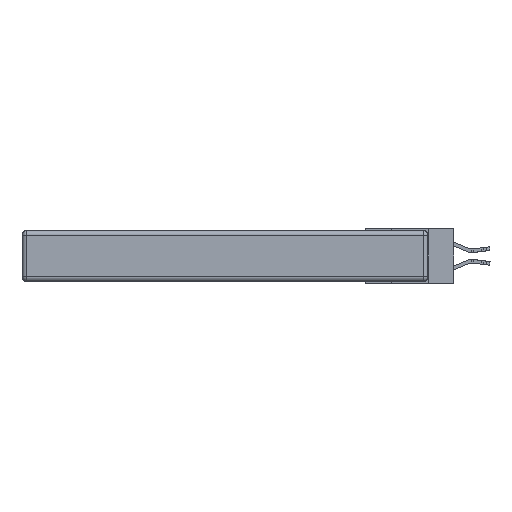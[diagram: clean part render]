
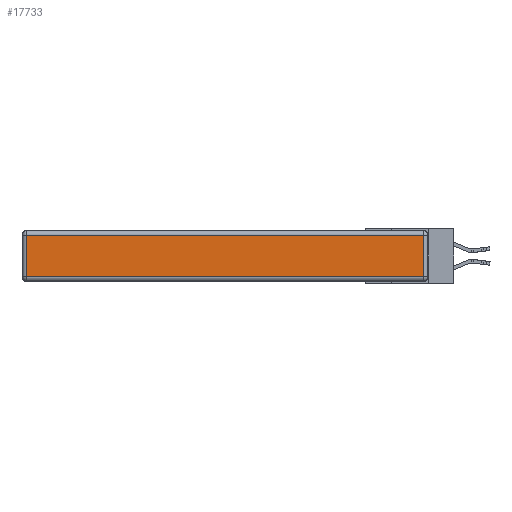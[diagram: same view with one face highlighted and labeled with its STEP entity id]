
A CAD part, left-side view. The second image highlights one B-rep face of the part: STEP entity #17733.
In plain terms, the highlighted planar face has unit normal (-1, 0, 0).
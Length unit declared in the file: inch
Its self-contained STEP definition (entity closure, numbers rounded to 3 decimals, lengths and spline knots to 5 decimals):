
#288 = LINE ( 'NONE', #23398, #34174 ) ;
#1447 = LINE ( 'NONE', #11361, #13348 ) ;
#2224 = PLANE ( 'NONE',  #32942 ) ;
#2473 = EDGE_CURVE ( 'NONE', #10716, #35085, #288, .T. ) ;
#3877 = CARTESIAN_POINT ( 'NONE',  ( 0., 2.72, -0.03 ) ) ;
#3889 = ORIENTED_EDGE ( 'NONE', *, *, #24011, .T. ) ;
#5048 = VECTOR ( 'NONE', #9613, 39.37008 ) ;
#6638 = CARTESIAN_POINT ( 'NONE',  ( 0., 0.03, -0.343 ) ) ;
#7925 = VERTEX_POINT ( 'NONE', #21688 ) ;
#8043 = VERTEX_POINT ( 'NONE', #25002 ) ;
#9613 = DIRECTION ( 'NONE',  ( 0., 0., 1. ) ) ;
#9906 = DIRECTION ( 'NONE',  ( 0., -1., 0. ) ) ;
#10716 = VERTEX_POINT ( 'NONE', #3877 ) ;
#10955 = FACE_OUTER_BOUND ( 'NONE', #35628, .T. ) ;
#11361 = CARTESIAN_POINT ( 'NONE',  ( 0., 2.75, -0.03 ) ) ;
#13348 = VECTOR ( 'NONE', #14070, 39.37008 ) ;
#13727 = ORIENTED_EDGE ( 'NONE', *, *, #20239, .T. ) ;
#14070 = DIRECTION ( 'NONE',  ( 0., 1., 0. ) ) ;
#15763 = DIRECTION ( 'NONE',  ( -1., 0., 0. ) ) ;
#17733 = ADVANCED_FACE ( 'NONE', ( #10955 ), #2224, .T. ) ;
#18973 = CARTESIAN_POINT ( 'NONE',  ( 0., 0., -0.343 ) ) ;
#20239 = EDGE_CURVE ( 'NONE', #7925, #10716, #1447, .T. ) ;
#21597 = EDGE_CURVE ( 'NONE', #35085, #8043, #23354, .T. ) ;
#21688 = CARTESIAN_POINT ( 'NONE',  ( 0., 0.03, -0.03 ) ) ;
#21885 = ORIENTED_EDGE ( 'NONE', *, *, #21597, .T. ) ;
#23354 = LINE ( 'NONE', #32181, #35647 ) ;
#23398 = CARTESIAN_POINT ( 'NONE',  ( 0., 2.72, -0.343 ) ) ;
#24011 = EDGE_CURVE ( 'NONE', #8043, #7925, #35017, .T. ) ;
#24137 = DIRECTION ( 'NONE',  ( 0., 0., 1. ) ) ;
#25002 = CARTESIAN_POINT ( 'NONE',  ( 0., 0.03, -0.313 ) ) ;
#25596 = DIRECTION ( 'NONE',  ( 0., 0., -1. ) ) ;
#29970 = ORIENTED_EDGE ( 'NONE', *, *, #2473, .T. ) ;
#32181 = CARTESIAN_POINT ( 'NONE',  ( 0., 0., -0.313 ) ) ;
#32942 = AXIS2_PLACEMENT_3D ( 'NONE', #18973, #15763, #24137 ) ;
#33662 = CARTESIAN_POINT ( 'NONE',  ( 0., 2.72, -0.313 ) ) ;
#34174 = VECTOR ( 'NONE', #25596, 39.37008 ) ;
#35017 = LINE ( 'NONE', #6638, #5048 ) ;
#35085 = VERTEX_POINT ( 'NONE', #33662 ) ;
#35628 = EDGE_LOOP ( 'NONE', ( #21885, #3889, #13727, #29970 ) ) ;
#35647 = VECTOR ( 'NONE', #9906, 39.37008 ) ;
